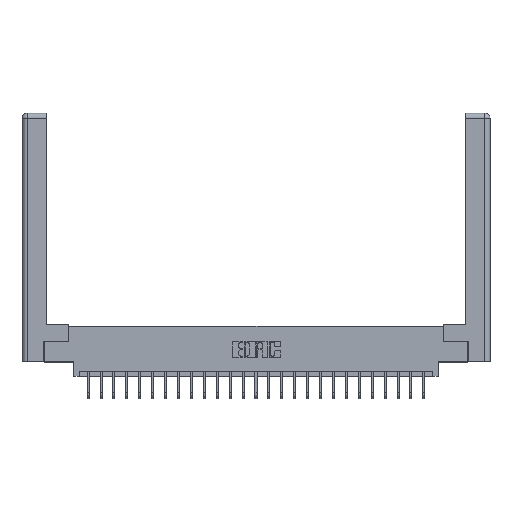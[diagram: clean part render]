
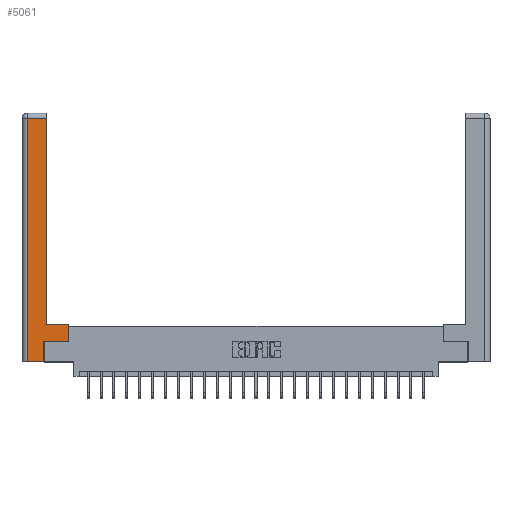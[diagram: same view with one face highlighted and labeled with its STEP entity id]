
A CAD part, top view. The second image highlights one B-rep face of the part: STEP entity #5061.
In plain terms, the highlighted planar face has unit normal (0, 0, 1).
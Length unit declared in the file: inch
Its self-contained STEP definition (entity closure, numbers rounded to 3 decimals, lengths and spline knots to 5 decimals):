
#38 = VECTOR ( 'NONE', #3180, 39.37008 ) ;
#236 = CARTESIAN_POINT ( 'NONE',  ( 0.565, 0.45, 0. ) ) ;
#621 = VERTEX_POINT ( 'NONE', #17602 ) ;
#791 = EDGE_CURVE ( 'NONE', #22597, #25389, #10589, .T. ) ;
#1013 = VECTOR ( 'NONE', #2445, 39.37008 ) ;
#1620 = EDGE_CURVE ( 'NONE', #8848, #621, #10871, .T. ) ;
#2445 = DIRECTION ( 'NONE',  ( 0., 1., 0. ) ) ;
#2487 = EDGE_CURVE ( 'NONE', #25389, #8298, #23136, .T. ) ;
#3180 = DIRECTION ( 'NONE',  ( 0., -1., 0. ) ) ;
#3925 = VECTOR ( 'NONE', #22386, 39.37008 ) ;
#4261 = DIRECTION ( 'NONE',  ( 1., 0., 0. ) ) ;
#4427 = CARTESIAN_POINT ( 'NONE',  ( 0.265, 0., 0. ) ) ;
#4532 = AXIS2_PLACEMENT_3D ( 'NONE', #10633, #16605, #20941 ) ;
#5061 = ADVANCED_FACE ( 'NONE', ( #26366 ), #12686, .F. ) ;
#5232 = VERTEX_POINT ( 'NONE', #9524 ) ;
#5560 = CARTESIAN_POINT ( 'NONE',  ( 0.265, 0.245, 0. ) ) ;
#5689 = EDGE_CURVE ( 'NONE', #8298, #9023, #23282, .T. ) ;
#5914 = LINE ( 'NONE', #21330, #14491 ) ;
#7112 = EDGE_CURVE ( 'NONE', #5232, #8848, #9112, .T. ) ;
#7940 = EDGE_CURVE ( 'NONE', #621, #22597, #17691, .T. ) ;
#8298 = VERTEX_POINT ( 'NONE', #19337 ) ;
#8848 = VERTEX_POINT ( 'NONE', #21749 ) ;
#8903 = ORIENTED_EDGE ( 'NONE', *, *, #2487, .T. ) ;
#8905 = DIRECTION ( 'NONE',  ( -1., 0., 0. ) ) ;
#9023 = VERTEX_POINT ( 'NONE', #13876 ) ;
#9112 = LINE ( 'NONE', #4427, #24732 ) ;
#9467 = CARTESIAN_POINT ( 'NONE',  ( 0.0615, 0., 0. ) ) ;
#9524 = CARTESIAN_POINT ( 'NONE',  ( 0.0615, 0., 0. ) ) ;
#9656 = CARTESIAN_POINT ( 'NONE',  ( 0.565, 0.45, 0. ) ) ;
#9767 = ORIENTED_EDGE ( 'NONE', *, *, #791, .T. ) ;
#9933 = EDGE_CURVE ( 'NONE', #25938, #5232, #21228, .T. ) ;
#10589 = LINE ( 'NONE', #236, #1013 ) ;
#10633 = CARTESIAN_POINT ( 'NONE',  ( 0., 0., 0. ) ) ;
#10871 = LINE ( 'NONE', #5560, #3925 ) ;
#11805 = CARTESIAN_POINT ( 'NONE',  ( 0.295, 3., 0. ) ) ;
#12686 = PLANE ( 'NONE',  #4532 ) ;
#13876 = CARTESIAN_POINT ( 'NONE',  ( 0.295, 2.94, 0. ) ) ;
#14491 = VECTOR ( 'NONE', #8905, 39.37008 ) ;
#16605 = DIRECTION ( 'NONE',  ( 0., 0., -1. ) ) ;
#17602 = CARTESIAN_POINT ( 'NONE',  ( 0.265, 0.245, 0. ) ) ;
#17636 = VECTOR ( 'NONE', #18407, 39.37008 ) ;
#17691 = LINE ( 'NONE', #25413, #24014 ) ;
#18407 = DIRECTION ( 'NONE',  ( 0., 1., 0. ) ) ;
#19147 = VECTOR ( 'NONE', #24018, 39.37008 ) ;
#19337 = CARTESIAN_POINT ( 'NONE',  ( 0.295, 0.45, 0. ) ) ;
#19583 = EDGE_CURVE ( 'NONE', #9023, #25938, #5914, .T. ) ;
#20513 = ORIENTED_EDGE ( 'NONE', *, *, #9933, .T. ) ;
#20602 = ORIENTED_EDGE ( 'NONE', *, *, #7112, .T. ) ;
#20918 = DIRECTION ( 'NONE',  ( 1., 0., 0. ) ) ;
#20941 = DIRECTION ( 'NONE',  ( -1., 0., 0. ) ) ;
#21228 = LINE ( 'NONE', #9467, #38 ) ;
#21330 = CARTESIAN_POINT ( 'NONE',  ( 0.0615, 2.94, 0. ) ) ;
#21734 = CARTESIAN_POINT ( 'NONE',  ( 0.0615, 2.94, 0. ) ) ;
#21749 = CARTESIAN_POINT ( 'NONE',  ( 0.265, 0., 0. ) ) ;
#22057 = CARTESIAN_POINT ( 'NONE',  ( 0.295, 0.45, 0. ) ) ;
#22386 = DIRECTION ( 'NONE',  ( 0., 1., 0. ) ) ;
#22597 = VERTEX_POINT ( 'NONE', #24395 ) ;
#23136 = LINE ( 'NONE', #22057, #19147 ) ;
#23282 = LINE ( 'NONE', #11805, #17636 ) ;
#23804 = ORIENTED_EDGE ( 'NONE', *, *, #5689, .T. ) ;
#24014 = VECTOR ( 'NONE', #4261, 39.37008 ) ;
#24018 = DIRECTION ( 'NONE',  ( -1., 0., 0. ) ) ;
#24395 = CARTESIAN_POINT ( 'NONE',  ( 0.565, 0.245, 0. ) ) ;
#24732 = VECTOR ( 'NONE', #20918, 39.37008 ) ;
#25056 = ORIENTED_EDGE ( 'NONE', *, *, #1620, .T. ) ;
#25389 = VERTEX_POINT ( 'NONE', #9656 ) ;
#25413 = CARTESIAN_POINT ( 'NONE',  ( 0.565, 0.245, 0. ) ) ;
#25938 = VERTEX_POINT ( 'NONE', #21734 ) ;
#26033 = ORIENTED_EDGE ( 'NONE', *, *, #7940, .T. ) ;
#26366 = FACE_OUTER_BOUND ( 'NONE', #26564, .T. ) ;
#26564 = EDGE_LOOP ( 'NONE', ( #23804, #27198, #20513, #20602, #25056, #26033, #9767, #8903 ) ) ;
#27198 = ORIENTED_EDGE ( 'NONE', *, *, #19583, .T. ) ;
